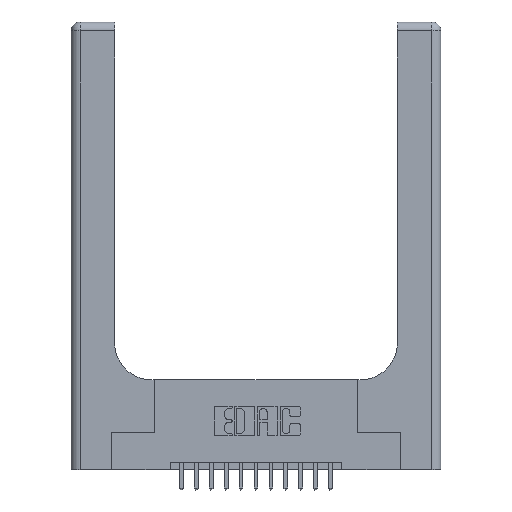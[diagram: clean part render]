
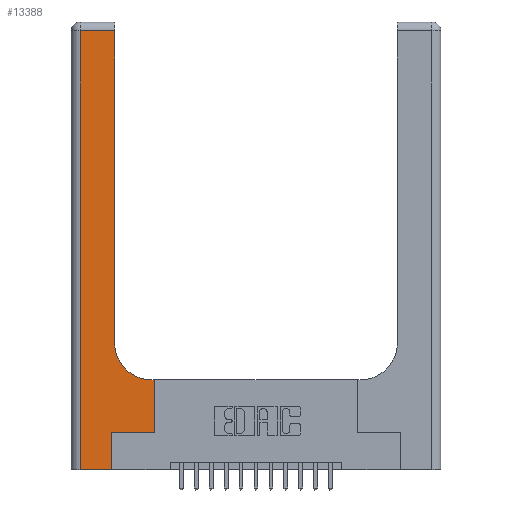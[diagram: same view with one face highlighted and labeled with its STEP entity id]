
A CAD part, top view. The second image highlights one B-rep face of the part: STEP entity #13388.
In plain terms, the highlighted planar face has unit normal (0, 0, 1).
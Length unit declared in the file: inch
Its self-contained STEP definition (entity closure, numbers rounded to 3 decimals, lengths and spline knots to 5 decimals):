
#218 = VERTEX_POINT ( 'NONE', #3522 ) ;
#271 = VERTEX_POINT ( 'NONE', #7796 ) ;
#678 = CARTESIAN_POINT ( 'NONE',  ( 0., 2.94, 0.37 ) ) ;
#686 = CIRCLE ( 'NONE', #9204, 0.25 ) ;
#815 = CARTESIAN_POINT ( 'NONE',  ( 0., 3., 0.37 ) ) ;
#1647 = EDGE_CURVE ( 'NONE', #16240, #218, #3844, .T. ) ;
#1881 = CARTESIAN_POINT ( 'NONE',  ( 0.269, 0.25, 0.37 ) ) ;
#2032 = DIRECTION ( 'NONE',  ( 0., 1., 0. ) ) ;
#2508 = VERTEX_POINT ( 'NONE', #5099 ) ;
#2741 = LINE ( 'NONE', #10314, #6023 ) ;
#2979 = EDGE_CURVE ( 'NONE', #2508, #16240, #8466, .T. ) ;
#3278 = ORIENTED_EDGE ( 'NONE', *, *, #17094, .T. ) ;
#3518 = ORIENTED_EDGE ( 'NONE', *, *, #17942, .T. ) ;
#3522 = CARTESIAN_POINT ( 'NONE',  ( 0.5415, 0.6, 0.37 ) ) ;
#3844 = LINE ( 'NONE', #16133, #7751 ) ;
#4324 = DIRECTION ( 'NONE',  ( 0., 1., 0. ) ) ;
#4744 = ORIENTED_EDGE ( 'NONE', *, *, #14518, .T. ) ;
#4862 = DIRECTION ( 'NONE',  ( 0., 1., 0. ) ) ;
#4998 = ORIENTED_EDGE ( 'NONE', *, *, #15341, .T. ) ;
#5099 = CARTESIAN_POINT ( 'NONE',  ( 0.5585, 0.25, 0.37 ) ) ;
#5101 = VECTOR ( 'NONE', #5468, 39.37008 ) ;
#5468 = DIRECTION ( 'NONE',  ( 0., -1., 0. ) ) ;
#5510 = VECTOR ( 'NONE', #4324, 39.37008 ) ;
#6023 = VECTOR ( 'NONE', #4862, 39.37008 ) ;
#6100 = VECTOR ( 'NONE', #2032, 39.37008 ) ;
#6431 = CARTESIAN_POINT ( 'NONE',  ( 0.5585, 0.6, 0.37 ) ) ;
#7073 = CARTESIAN_POINT ( 'NONE',  ( 0.5415, 0.85, 0.37 ) ) ;
#7751 = VECTOR ( 'NONE', #17576, 39.37008 ) ;
#7796 = CARTESIAN_POINT ( 'NONE',  ( 0.2915, 2.94, 0.37 ) ) ;
#7822 = LINE ( 'NONE', #8250, #14784 ) ;
#7960 = VERTEX_POINT ( 'NONE', #1881 ) ;
#8076 = VERTEX_POINT ( 'NONE', #11352 ) ;
#8250 = CARTESIAN_POINT ( 'NONE',  ( 0.269, 0.25, 0.37 ) ) ;
#8295 = EDGE_CURVE ( 'NONE', #8076, #14097, #15731, .T. ) ;
#8441 = CARTESIAN_POINT ( 'NONE',  ( 0.269, 0., 0.37 ) ) ;
#8466 = LINE ( 'NONE', #15868, #6100 ) ;
#8503 = PLANE ( 'NONE',  #15594 ) ;
#9204 = AXIS2_PLACEMENT_3D ( 'NONE', #7073, #13887, #16624 ) ;
#9637 = ORIENTED_EDGE ( 'NONE', *, *, #10400, .T. ) ;
#9727 = ORIENTED_EDGE ( 'NONE', *, *, #1647, .T. ) ;
#9887 = DIRECTION ( 'NONE',  ( 1., 0., 0. ) ) ;
#10085 = LINE ( 'NONE', #10906, #5101 ) ;
#10314 = CARTESIAN_POINT ( 'NONE',  ( 0.2915, 3., 0.37 ) ) ;
#10321 = LINE ( 'NONE', #678, #17084 ) ;
#10400 = EDGE_CURVE ( 'NONE', #7960, #2508, #7822, .T. ) ;
#10436 = DIRECTION ( 'NONE',  ( -1., 0., 0. ) ) ;
#10906 = CARTESIAN_POINT ( 'NONE',  ( 0.06, 3., 0.37 ) ) ;
#11054 = ORIENTED_EDGE ( 'NONE', *, *, #2979, .T. ) ;
#11135 = LINE ( 'NONE', #8441, #5510 ) ;
#11141 = ORIENTED_EDGE ( 'NONE', *, *, #8295, .T. ) ;
#11271 = CARTESIAN_POINT ( 'NONE',  ( 0.269, 0., 0.37 ) ) ;
#11352 = CARTESIAN_POINT ( 'NONE',  ( 0.06, 0., 0.37 ) ) ;
#11501 = CARTESIAN_POINT ( 'NONE',  ( 0.2915, 0.85, 0.37 ) ) ;
#11919 = VERTEX_POINT ( 'NONE', #17541 ) ;
#12207 = DIRECTION ( 'NONE',  ( 1., 0., 0. ) ) ;
#12358 = EDGE_CURVE ( 'NONE', #15989, #271, #2741, .T. ) ;
#12643 = VECTOR ( 'NONE', #12207, 39.37008 ) ;
#13218 = DIRECTION ( 'NONE',  ( 0., 0., -1. ) ) ;
#13388 = ADVANCED_FACE ( 'NONE', ( #17093 ), #8503, .F. ) ;
#13887 = DIRECTION ( 'NONE',  ( 0., 0., -1. ) ) ;
#14097 = VERTEX_POINT ( 'NONE', #11271 ) ;
#14518 = EDGE_CURVE ( 'NONE', #11919, #8076, #10085, .T. ) ;
#14741 = DIRECTION ( 'NONE',  ( -1., 0., 0. ) ) ;
#14784 = VECTOR ( 'NONE', #9887, 39.37008 ) ;
#15113 = CARTESIAN_POINT ( 'NONE',  ( 0., 0., 0.37 ) ) ;
#15341 = EDGE_CURVE ( 'NONE', #14097, #7960, #11135, .T. ) ;
#15594 = AXIS2_PLACEMENT_3D ( 'NONE', #815, #13218, #14741 ) ;
#15693 = EDGE_LOOP ( 'NONE', ( #16571, #3278, #4744, #11141, #4998, #9637, #11054, #9727, #3518 ) ) ;
#15731 = LINE ( 'NONE', #15113, #12643 ) ;
#15868 = CARTESIAN_POINT ( 'NONE',  ( 0.5585, 0.25, 0.37 ) ) ;
#15989 = VERTEX_POINT ( 'NONE', #11501 ) ;
#16133 = CARTESIAN_POINT ( 'NONE',  ( 0.2915, 0.6, 0.37 ) ) ;
#16240 = VERTEX_POINT ( 'NONE', #6431 ) ;
#16571 = ORIENTED_EDGE ( 'NONE', *, *, #12358, .T. ) ;
#16624 = DIRECTION ( 'NONE',  ( 1., 0., 0. ) ) ;
#17084 = VECTOR ( 'NONE', #10436, 39.37008 ) ;
#17093 = FACE_OUTER_BOUND ( 'NONE', #15693, .T. ) ;
#17094 = EDGE_CURVE ( 'NONE', #271, #11919, #10321, .T. ) ;
#17541 = CARTESIAN_POINT ( 'NONE',  ( 0.06, 2.94, 0.37 ) ) ;
#17576 = DIRECTION ( 'NONE',  ( -1., 0., 0. ) ) ;
#17942 = EDGE_CURVE ( 'NONE', #218, #15989, #686, .T. ) ;
